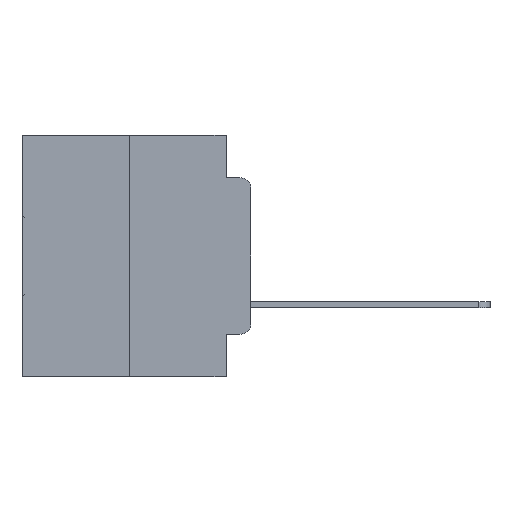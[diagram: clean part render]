
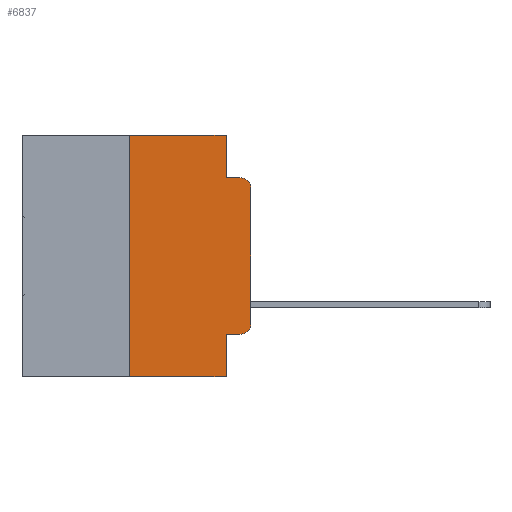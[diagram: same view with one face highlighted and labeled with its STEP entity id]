
A CAD part, left-side view. The second image highlights one B-rep face of the part: STEP entity #6837.
In plain terms, the highlighted planar face has unit normal (-1, 0, 0).
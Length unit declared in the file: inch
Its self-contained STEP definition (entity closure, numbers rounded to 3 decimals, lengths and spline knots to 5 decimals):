
#805 = VERTEX_POINT ( 'NONE', #13865 ) ;
#1132 = AXIS2_PLACEMENT_3D ( 'NONE', #18802, #14065, #30343 ) ;
#1277 = CARTESIAN_POINT ( 'NONE',  ( 0., 0.051, -0.5 ) ) ;
#2744 = EDGE_CURVE ( 'NONE', #805, #26618, #30457, .T. ) ;
#3386 = VERTEX_POINT ( 'NONE', #7626 ) ;
#3433 = DIRECTION ( 'NONE',  ( 0., -1., 0. ) ) ;
#3462 = EDGE_CURVE ( 'NONE', #3386, #21519, #3597, .T. ) ;
#3562 = VERTEX_POINT ( 'NONE', #23518 ) ;
#3595 = CARTESIAN_POINT ( 'NONE',  ( 0., 0.051, 0. ) ) ;
#3597 = LINE ( 'NONE', #28984, #28617 ) ;
#3788 = AXIS2_PLACEMENT_3D ( 'NONE', #5628, #22849, #8245 ) ;
#4852 = LINE ( 'NONE', #10888, #18938 ) ;
#4962 = ORIENTED_EDGE ( 'NONE', *, *, #28846, .T. ) ;
#5416 = ORIENTED_EDGE ( 'NONE', *, *, #24300, .T. ) ;
#5601 = CARTESIAN_POINT ( 'NONE',  ( 0., 0., -0.3915 ) ) ;
#5628 = CARTESIAN_POINT ( 'NONE',  ( 0., 0.02, -0.3915 ) ) ;
#5971 = ORIENTED_EDGE ( 'NONE', *, *, #9796, .F. ) ;
#6280 = CARTESIAN_POINT ( 'NONE',  ( 0., 0.25, -0.5 ) ) ;
#6448 = VERTEX_POINT ( 'NONE', #17050 ) ;
#6837 = ADVANCED_FACE ( 'NONE', ( #28314 ), #11575, .F. ) ;
#7000 = ORIENTED_EDGE ( 'NONE', *, *, #2744, .F. ) ;
#7245 = VERTEX_POINT ( 'NONE', #25501 ) ;
#7626 = CARTESIAN_POINT ( 'NONE',  ( 0., 0.051, -0.4115 ) ) ;
#7843 = CARTESIAN_POINT ( 'NONE',  ( 0., 0., 0. ) ) ;
#8031 = LINE ( 'NONE', #7843, #27188 ) ;
#8245 = DIRECTION ( 'NONE',  ( 0., 0., -1. ) ) ;
#9021 = DIRECTION ( 'NONE',  ( -1., 0., 0. ) ) ;
#9360 = DIRECTION ( 'NONE',  ( 0., 0., 1. ) ) ;
#9416 = ORIENTED_EDGE ( 'NONE', *, *, #17573, .F. ) ;
#9796 = EDGE_CURVE ( 'NONE', #26618, #6448, #20679, .T. ) ;
#9983 = ORIENTED_EDGE ( 'NONE', *, *, #23347, .F. ) ;
#10346 = ORIENTED_EDGE ( 'NONE', *, *, #28550, .T. ) ;
#10594 = DIRECTION ( 'NONE',  ( 0., 0., -1. ) ) ;
#10755 = EDGE_LOOP ( 'NONE', ( #4962, #5416, #5971, #7000, #9416, #9983, #10346, #10837, #11364, #11753 ) ) ;
#10837 = ORIENTED_EDGE ( 'NONE', *, *, #3462, .F. ) ;
#10888 = CARTESIAN_POINT ( 'NONE',  ( 0., 0.473, 0. ) ) ;
#11364 = ORIENTED_EDGE ( 'NONE', *, *, #28471, .T. ) ;
#11575 = PLANE ( 'NONE',  #1132 ) ;
#11753 = ORIENTED_EDGE ( 'NONE', *, *, #20815, .T. ) ;
#13304 = VECTOR ( 'NONE', #17383, 39.37008 ) ;
#13865 = CARTESIAN_POINT ( 'NONE',  ( 0., 0.051, 0. ) ) ;
#14065 = DIRECTION ( 'NONE',  ( 1., 0., 0. ) ) ;
#14188 = CARTESIAN_POINT ( 'NONE',  ( 0., 0.051, -0.4115 ) ) ;
#15852 = VERTEX_POINT ( 'NONE', #5601 ) ;
#16674 = LINE ( 'NONE', #28361, #22211 ) ;
#17050 = CARTESIAN_POINT ( 'NONE',  ( 0., 0.02, -0.0885 ) ) ;
#17383 = DIRECTION ( 'NONE',  ( 0., 0., -1. ) ) ;
#17573 = EDGE_CURVE ( 'NONE', #24474, #805, #4852, .T. ) ;
#18548 = AXIS2_PLACEMENT_3D ( 'NONE', #23498, #9021, #25805 ) ;
#18802 = CARTESIAN_POINT ( 'NONE',  ( 0., 0.473, 0. ) ) ;
#18938 = VECTOR ( 'NONE', #27452, 39.37008 ) ;
#19071 = CIRCLE ( 'NONE', #18548, 0.02 ) ;
#19291 = CARTESIAN_POINT ( 'NONE',  ( 0., 0.25, 0. ) ) ;
#20679 = LINE ( 'NONE', #20916, #27500 ) ;
#20815 = EDGE_CURVE ( 'NONE', #7245, #15852, #28343, .T. ) ;
#20916 = CARTESIAN_POINT ( 'NONE',  ( 0., 0.051, -0.0885 ) ) ;
#21519 = VERTEX_POINT ( 'NONE', #1277 ) ;
#21613 = CARTESIAN_POINT ( 'NONE',  ( 0., 0.25, 0. ) ) ;
#22211 = VECTOR ( 'NONE', #26208, 39.37008 ) ;
#22441 = LINE ( 'NONE', #21613, #27062 ) ;
#22849 = DIRECTION ( 'NONE',  ( -1., 0., 0. ) ) ;
#23347 = EDGE_CURVE ( 'NONE', #29133, #24474, #22441, .T. ) ;
#23498 = CARTESIAN_POINT ( 'NONE',  ( 0., 0.02, -0.1085 ) ) ;
#23518 = CARTESIAN_POINT ( 'NONE',  ( 0., 0., -0.1085 ) ) ;
#23645 = VECTOR ( 'NONE', #28176, 39.37008 ) ;
#24300 = EDGE_CURVE ( 'NONE', #3562, #6448, #19071, .T. ) ;
#24474 = VERTEX_POINT ( 'NONE', #19291 ) ;
#25501 = CARTESIAN_POINT ( 'NONE',  ( 0., 0.02, -0.4115 ) ) ;
#25805 = DIRECTION ( 'NONE',  ( 0., 0., -1. ) ) ;
#26208 = DIRECTION ( 'NONE',  ( 0., -1., 0. ) ) ;
#26618 = VERTEX_POINT ( 'NONE', #27154 ) ;
#27062 = VECTOR ( 'NONE', #9360, 39.37008 ) ;
#27154 = CARTESIAN_POINT ( 'NONE',  ( 0., 0.051, -0.0885 ) ) ;
#27188 = VECTOR ( 'NONE', #31570, 39.37008 ) ;
#27452 = DIRECTION ( 'NONE',  ( 0., -1., 0. ) ) ;
#27500 = VECTOR ( 'NONE', #3433, 39.37008 ) ;
#28176 = DIRECTION ( 'NONE',  ( 0., -1., 0. ) ) ;
#28314 = FACE_OUTER_BOUND ( 'NONE', #10755, .T. ) ;
#28343 = CIRCLE ( 'NONE', #3788, 0.02 ) ;
#28361 = CARTESIAN_POINT ( 'NONE',  ( 0., 0.473, -0.5 ) ) ;
#28471 = EDGE_CURVE ( 'NONE', #3386, #7245, #29678, .T. ) ;
#28550 = EDGE_CURVE ( 'NONE', #29133, #21519, #16674, .T. ) ;
#28617 = VECTOR ( 'NONE', #10594, 39.37008 ) ;
#28846 = EDGE_CURVE ( 'NONE', #15852, #3562, #8031, .T. ) ;
#28984 = CARTESIAN_POINT ( 'NONE',  ( 0., 0.051, 0. ) ) ;
#29133 = VERTEX_POINT ( 'NONE', #6280 ) ;
#29678 = LINE ( 'NONE', #14188, #23645 ) ;
#30343 = DIRECTION ( 'NONE',  ( 0., 0., -1. ) ) ;
#30457 = LINE ( 'NONE', #3595, #13304 ) ;
#31570 = DIRECTION ( 'NONE',  ( 0., 0., 1. ) ) ;
